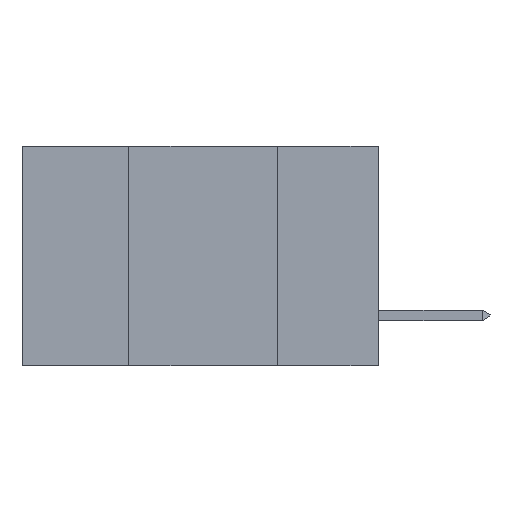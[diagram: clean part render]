
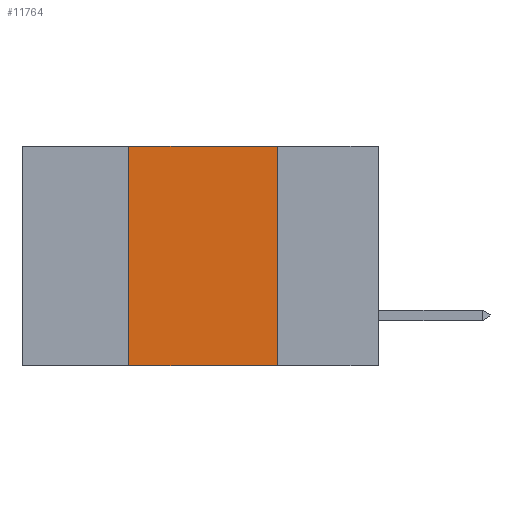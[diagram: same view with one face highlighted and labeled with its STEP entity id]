
A CAD part, left-side view. The second image highlights one B-rep face of the part: STEP entity #11764.
In plain terms, the highlighted planar face has unit normal (-1, 0, 0).
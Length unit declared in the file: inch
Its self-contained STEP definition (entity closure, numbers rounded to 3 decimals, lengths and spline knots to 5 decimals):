
#227 = CARTESIAN_POINT ( 'NONE',  ( 0., 0.6, -0.37 ) ) ;
#708 = EDGE_CURVE ( 'NONE', #14646, #15113, #14586, .T. ) ;
#1179 = DIRECTION ( 'NONE',  ( 1., 0., 0. ) ) ;
#1821 = VECTOR ( 'NONE', #13945, 39.37008 ) ;
#1882 = CARTESIAN_POINT ( 'NONE',  ( 0., 0.17, 0. ) ) ;
#2227 = DIRECTION ( 'NONE',  ( 0., 0., -1. ) ) ;
#2312 = AXIS2_PLACEMENT_3D ( 'NONE', #3080, #1179, #14567 ) ;
#2813 = ORIENTED_EDGE ( 'NONE', *, *, #15418, .F. ) ;
#3080 = CARTESIAN_POINT ( 'NONE',  ( 0., 0.6, 0. ) ) ;
#6801 = VECTOR ( 'NONE', #11746, 39.37008 ) ;
#9372 = CARTESIAN_POINT ( 'NONE',  ( 0., 0.42, 0. ) ) ;
#9798 = EDGE_LOOP ( 'NONE', ( #22943, #23986, #2813, #20026 ) ) ;
#10391 = LINE ( 'NONE', #9372, #18452 ) ;
#10797 = CARTESIAN_POINT ( 'NONE',  ( 0., 0.17, 0. ) ) ;
#11746 = DIRECTION ( 'NONE',  ( 0., -1., 0. ) ) ;
#11764 = ADVANCED_FACE ( 'NONE', ( #22358 ), #24252, .F. ) ;
#12137 = CARTESIAN_POINT ( 'NONE',  ( 0., 0.42, 0. ) ) ;
#13346 = CARTESIAN_POINT ( 'NONE',  ( 0., 0.42, -0.37 ) ) ;
#13945 = DIRECTION ( 'NONE',  ( 0., -1., 0. ) ) ;
#14511 = LINE ( 'NONE', #19430, #6801 ) ;
#14567 = DIRECTION ( 'NONE',  ( 0., 0., -1. ) ) ;
#14586 = LINE ( 'NONE', #227, #1821 ) ;
#14646 = VERTEX_POINT ( 'NONE', #13346 ) ;
#15113 = VERTEX_POINT ( 'NONE', #20207 ) ;
#15418 = EDGE_CURVE ( 'NONE', #14646, #19981, #10391, .T. ) ;
#16868 = VERTEX_POINT ( 'NONE', #10797 ) ;
#18452 = VECTOR ( 'NONE', #22695, 39.37008 ) ;
#18721 = EDGE_CURVE ( 'NONE', #16868, #15113, #18910, .T. ) ;
#18910 = LINE ( 'NONE', #1882, #21296 ) ;
#19430 = CARTESIAN_POINT ( 'NONE',  ( 0., 0.6, 0. ) ) ;
#19981 = VERTEX_POINT ( 'NONE', #12137 ) ;
#20026 = ORIENTED_EDGE ( 'NONE', *, *, #708, .T. ) ;
#20207 = CARTESIAN_POINT ( 'NONE',  ( 0., 0.17, -0.37 ) ) ;
#20615 = EDGE_CURVE ( 'NONE', #19981, #16868, #14511, .T. ) ;
#21296 = VECTOR ( 'NONE', #2227, 39.37008 ) ;
#22358 = FACE_OUTER_BOUND ( 'NONE', #9798, .T. ) ;
#22695 = DIRECTION ( 'NONE',  ( 0., 0., 1. ) ) ;
#22943 = ORIENTED_EDGE ( 'NONE', *, *, #18721, .F. ) ;
#23986 = ORIENTED_EDGE ( 'NONE', *, *, #20615, .F. ) ;
#24252 = PLANE ( 'NONE',  #2312 ) ;
